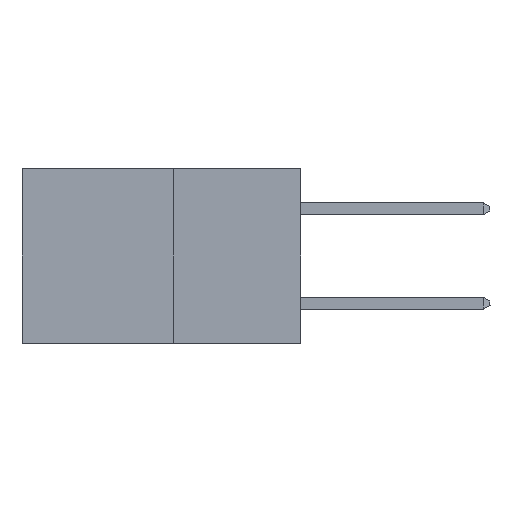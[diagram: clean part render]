
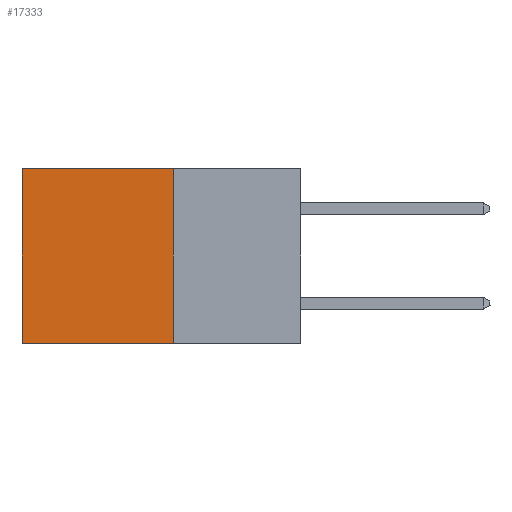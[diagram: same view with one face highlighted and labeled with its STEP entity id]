
A CAD part, left-side view. The second image highlights one B-rep face of the part: STEP entity #17333.
In plain terms, the highlighted planar face has unit normal (-1, 0, 0).
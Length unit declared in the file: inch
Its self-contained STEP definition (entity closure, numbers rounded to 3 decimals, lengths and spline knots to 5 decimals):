
#160 = DIRECTION ( 'NONE',  ( 0., 0., -1. ) ) ;
#196 = CARTESIAN_POINT ( 'NONE',  ( 0.277, 0.27, 0. ) ) ;
#796 = DIRECTION ( 'NONE',  ( 0., 0., -1. ) ) ;
#1005 = LINE ( 'NONE', #1499, #7999 ) ;
#1275 = DIRECTION ( 'NONE',  ( 0., 1., 0. ) ) ;
#1499 = CARTESIAN_POINT ( 'NONE',  ( 0.277, 0.59, -0.37 ) ) ;
#1848 = LINE ( 'NONE', #8521, #5576 ) ;
#3913 = FACE_OUTER_BOUND ( 'NONE', #5851, .T. ) ;
#4413 = CARTESIAN_POINT ( 'NONE',  ( 0.277, 0.27, -0.37 ) ) ;
#4757 = EDGE_CURVE ( 'NONE', #11054, #6096, #1848, .T. ) ;
#5576 = VECTOR ( 'NONE', #8489, 39.37008 ) ;
#5709 = DIRECTION ( 'NONE',  ( 0., 0., -1. ) ) ;
#5851 = EDGE_LOOP ( 'NONE', ( #12622, #12915, #14053, #15312 ) ) ;
#6096 = VERTEX_POINT ( 'NONE', #7661 ) ;
#6853 = LINE ( 'NONE', #7753, #13699 ) ;
#7661 = CARTESIAN_POINT ( 'NONE',  ( 0.277, 0.59, 0. ) ) ;
#7712 = LINE ( 'NONE', #17573, #14545 ) ;
#7753 = CARTESIAN_POINT ( 'NONE',  ( 0.277, 0.27, -0.37 ) ) ;
#7999 = VECTOR ( 'NONE', #5709, 39.37008 ) ;
#8489 = DIRECTION ( 'NONE',  ( 0., 1., 0. ) ) ;
#8521 = CARTESIAN_POINT ( 'NONE',  ( 0.277, 0.27, 0. ) ) ;
#8562 = DIRECTION ( 'NONE',  ( 1., 0., 0. ) ) ;
#10789 = CARTESIAN_POINT ( 'NONE',  ( 0.277, 0.27, -0.37 ) ) ;
#11054 = VERTEX_POINT ( 'NONE', #196 ) ;
#12150 = VERTEX_POINT ( 'NONE', #10789 ) ;
#12492 = VERTEX_POINT ( 'NONE', #13041 ) ;
#12622 = ORIENTED_EDGE ( 'NONE', *, *, #17286, .T. ) ;
#12915 = ORIENTED_EDGE ( 'NONE', *, *, #13029, .F. ) ;
#13029 = EDGE_CURVE ( 'NONE', #12150, #12492, #7712, .T. ) ;
#13041 = CARTESIAN_POINT ( 'NONE',  ( 0.277, 0.59, -0.37 ) ) ;
#13699 = VECTOR ( 'NONE', #796, 39.37008 ) ;
#14053 = ORIENTED_EDGE ( 'NONE', *, *, #14196, .F. ) ;
#14196 = EDGE_CURVE ( 'NONE', #11054, #12150, #6853, .T. ) ;
#14545 = VECTOR ( 'NONE', #1275, 39.37008 ) ;
#15312 = ORIENTED_EDGE ( 'NONE', *, *, #4757, .T. ) ;
#16167 = AXIS2_PLACEMENT_3D ( 'NONE', #4413, #8562, #160 ) ;
#16620 = PLANE ( 'NONE',  #16167 ) ;
#17286 = EDGE_CURVE ( 'NONE', #6096, #12492, #1005, .T. ) ;
#17333 = ADVANCED_FACE ( 'NONE', ( #3913 ), #16620, .F. ) ;
#17573 = CARTESIAN_POINT ( 'NONE',  ( 0.277, 0.27, -0.37 ) ) ;
